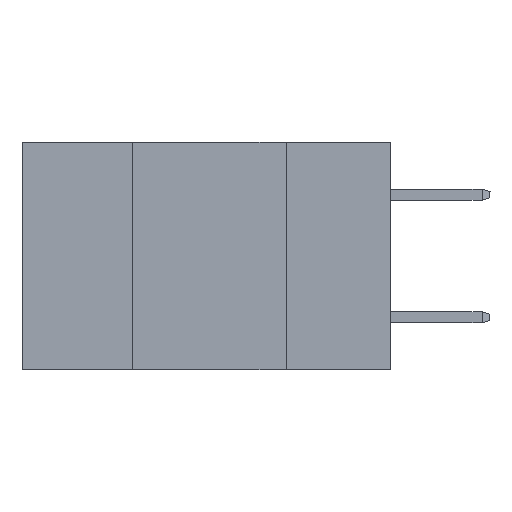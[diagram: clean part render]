
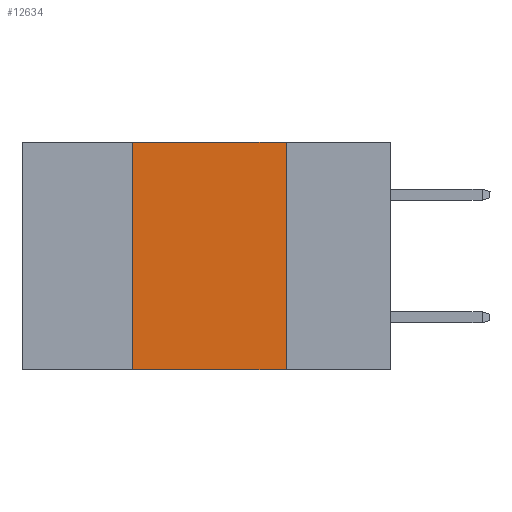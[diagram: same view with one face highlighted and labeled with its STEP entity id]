
A CAD part, left-side view. The second image highlights one B-rep face of the part: STEP entity #12634.
In plain terms, the highlighted planar face has unit normal (-1, 0, 0).
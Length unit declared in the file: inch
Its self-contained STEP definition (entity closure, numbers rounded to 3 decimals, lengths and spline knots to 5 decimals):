
#2874 = CARTESIAN_POINT ( 'NONE',  ( 0., 0.6, -0.37 ) ) ;
#3496 = ORIENTED_EDGE ( 'NONE', *, *, #22805, .F. ) ;
#4107 = LINE ( 'NONE', #22291, #20184 ) ;
#4403 = VERTEX_POINT ( 'NONE', #6154 ) ;
#4786 = EDGE_CURVE ( 'NONE', #4403, #21924, #7329, .T. ) ;
#5484 = VECTOR ( 'NONE', #7389, 39.37008 ) ;
#5702 = DIRECTION ( 'NONE',  ( 1., 0., 0. ) ) ;
#5929 = CARTESIAN_POINT ( 'NONE',  ( 0., 0.42, 0. ) ) ;
#6154 = CARTESIAN_POINT ( 'NONE',  ( 0., 0.42, -0.37 ) ) ;
#6426 = DIRECTION ( 'NONE',  ( 0., 0., 1. ) ) ;
#7329 = LINE ( 'NONE', #2874, #25241 ) ;
#7389 = DIRECTION ( 'NONE',  ( 0., 0., -1. ) ) ;
#7908 = DIRECTION ( 'NONE',  ( 0., -1., 0. ) ) ;
#8166 = CARTESIAN_POINT ( 'NONE',  ( 0., 0.17, 0. ) ) ;
#8607 = CARTESIAN_POINT ( 'NONE',  ( 0., 0.17, -0.37 ) ) ;
#11568 = ORIENTED_EDGE ( 'NONE', *, *, #4786, .T. ) ;
#11877 = FACE_OUTER_BOUND ( 'NONE', #19103, .T. ) ;
#12093 = VECTOR ( 'NONE', #6426, 39.37008 ) ;
#12310 = ORIENTED_EDGE ( 'NONE', *, *, #25268, .F. ) ;
#12634 = ADVANCED_FACE ( 'NONE', ( #11877 ), #25690, .F. ) ;
#13458 = CARTESIAN_POINT ( 'NONE',  ( 0., 0.42, 0. ) ) ;
#13808 = AXIS2_PLACEMENT_3D ( 'NONE', #23606, #5702, #15905 ) ;
#14495 = ORIENTED_EDGE ( 'NONE', *, *, #16876, .F. ) ;
#15234 = CARTESIAN_POINT ( 'NONE',  ( 0., 0.17, 0. ) ) ;
#15905 = DIRECTION ( 'NONE',  ( 0., 0., -1. ) ) ;
#16876 = EDGE_CURVE ( 'NONE', #20395, #16998, #4107, .T. ) ;
#16998 = VERTEX_POINT ( 'NONE', #8166 ) ;
#17276 = DIRECTION ( 'NONE',  ( 0., -1., 0. ) ) ;
#19103 = EDGE_LOOP ( 'NONE', ( #12310, #14495, #3496, #11568 ) ) ;
#20184 = VECTOR ( 'NONE', #7908, 39.37008 ) ;
#20395 = VERTEX_POINT ( 'NONE', #13458 ) ;
#21924 = VERTEX_POINT ( 'NONE', #8607 ) ;
#22291 = CARTESIAN_POINT ( 'NONE',  ( 0., 0.6, 0. ) ) ;
#22805 = EDGE_CURVE ( 'NONE', #4403, #20395, #23966, .T. ) ;
#23606 = CARTESIAN_POINT ( 'NONE',  ( 0., 0.6, 0. ) ) ;
#23718 = LINE ( 'NONE', #15234, #5484 ) ;
#23966 = LINE ( 'NONE', #5929, #12093 ) ;
#25241 = VECTOR ( 'NONE', #17276, 39.37008 ) ;
#25268 = EDGE_CURVE ( 'NONE', #16998, #21924, #23718, .T. ) ;
#25690 = PLANE ( 'NONE',  #13808 ) ;
